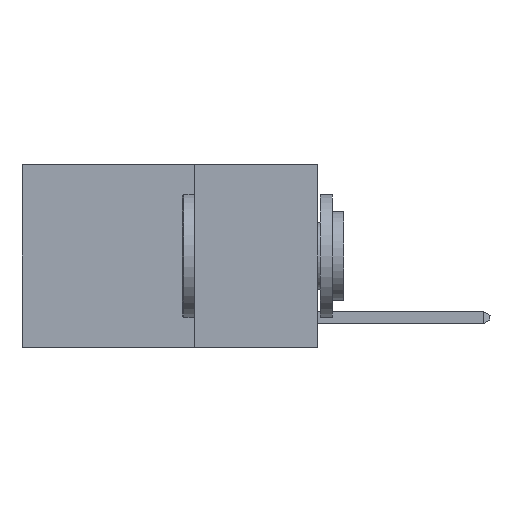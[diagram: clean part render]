
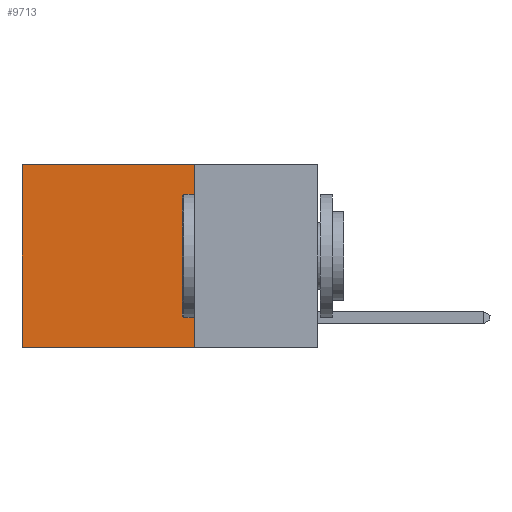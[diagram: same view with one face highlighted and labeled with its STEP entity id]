
A CAD part, left-side view. The second image highlights one B-rep face of the part: STEP entity #9713.
In plain terms, the highlighted planar face has unit normal (-1, 0, 0).
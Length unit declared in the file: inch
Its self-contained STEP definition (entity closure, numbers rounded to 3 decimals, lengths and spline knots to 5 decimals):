
#616 = AXIS2_PLACEMENT_3D ( 'NONE', #2461, #2775, #18488 ) ;
#1270 = LINE ( 'NONE', #4651, #2234 ) ;
#1978 = CARTESIAN_POINT ( 'NONE',  ( 0.2625, 0.25, 0. ) ) ;
#2234 = VECTOR ( 'NONE', #18316, 39.37008 ) ;
#2461 = CARTESIAN_POINT ( 'NONE',  ( 0.2625, 0.25, 0. ) ) ;
#2775 = DIRECTION ( 'NONE',  ( 1., 0., 0. ) ) ;
#2985 = EDGE_CURVE ( 'NONE', #11646, #14624, #1270, .T. ) ;
#4651 = CARTESIAN_POINT ( 'NONE',  ( 0.2625, 0.25, -0.37 ) ) ;
#5579 = EDGE_CURVE ( 'NONE', #16664, #14624, #9724, .T. ) ;
#6061 = EDGE_CURVE ( 'NONE', #12747, #16664, #16942, .T. ) ;
#6949 = CARTESIAN_POINT ( 'NONE',  ( 0.2625, 0.6, 0. ) ) ;
#9713 = ADVANCED_FACE ( 'NONE', ( #21432 ), #18258, .F. ) ;
#9724 = LINE ( 'NONE', #11873, #17078 ) ;
#10866 = ORIENTED_EDGE ( 'NONE', *, *, #5579, .T. ) ;
#11197 = EDGE_LOOP ( 'NONE', ( #10866, #19118, #12728, #16231 ) ) ;
#11500 = CARTESIAN_POINT ( 'NONE',  ( 0.2625, 0.25, 0. ) ) ;
#11559 = EDGE_CURVE ( 'NONE', #12747, #11646, #19277, .T. ) ;
#11646 = VERTEX_POINT ( 'NONE', #21296 ) ;
#11873 = CARTESIAN_POINT ( 'NONE',  ( 0.2625, 0.6, 0. ) ) ;
#12362 = DIRECTION ( 'NONE',  ( 0., 0., -1. ) ) ;
#12728 = ORIENTED_EDGE ( 'NONE', *, *, #11559, .F. ) ;
#12747 = VERTEX_POINT ( 'NONE', #13193 ) ;
#13086 = DIRECTION ( 'NONE',  ( 0., 1., 0. ) ) ;
#13193 = CARTESIAN_POINT ( 'NONE',  ( 0.2625, 0.25, 0. ) ) ;
#13856 = VECTOR ( 'NONE', #12362, 39.37008 ) ;
#14624 = VERTEX_POINT ( 'NONE', #17462 ) ;
#15041 = DIRECTION ( 'NONE',  ( 0., 0., -1. ) ) ;
#16231 = ORIENTED_EDGE ( 'NONE', *, *, #6061, .T. ) ;
#16664 = VERTEX_POINT ( 'NONE', #6949 ) ;
#16730 = VECTOR ( 'NONE', #13086, 39.37008 ) ;
#16942 = LINE ( 'NONE', #11500, #16730 ) ;
#17078 = VECTOR ( 'NONE', #15041, 39.37008 ) ;
#17462 = CARTESIAN_POINT ( 'NONE',  ( 0.2625, 0.6, -0.37 ) ) ;
#18258 = PLANE ( 'NONE',  #616 ) ;
#18316 = DIRECTION ( 'NONE',  ( 0., 1., 0. ) ) ;
#18488 = DIRECTION ( 'NONE',  ( 0., 0., -1. ) ) ;
#19118 = ORIENTED_EDGE ( 'NONE', *, *, #2985, .F. ) ;
#19277 = LINE ( 'NONE', #1978, #13856 ) ;
#21296 = CARTESIAN_POINT ( 'NONE',  ( 0.2625, 0.25, -0.37 ) ) ;
#21432 = FACE_OUTER_BOUND ( 'NONE', #11197, .T. ) ;
